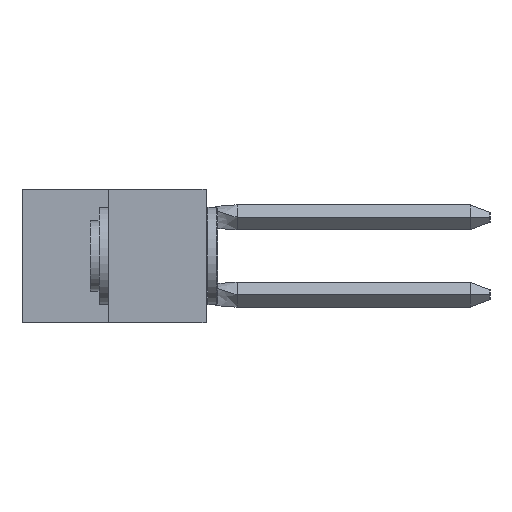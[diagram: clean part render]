
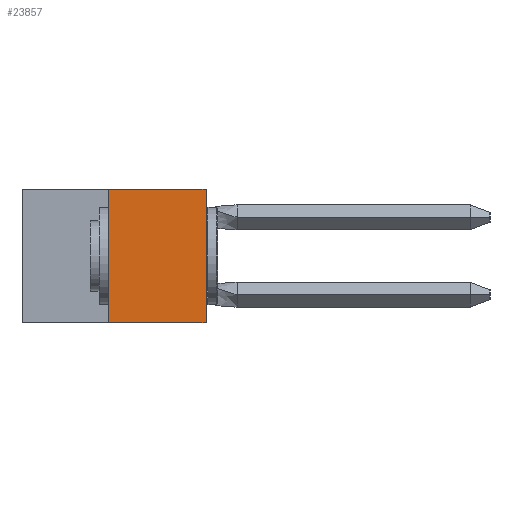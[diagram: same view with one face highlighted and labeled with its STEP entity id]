
A CAD part, left-side view. The second image highlights one B-rep face of the part: STEP entity #23857.
In plain terms, the highlighted planar face has unit normal (-1, 0, 0).
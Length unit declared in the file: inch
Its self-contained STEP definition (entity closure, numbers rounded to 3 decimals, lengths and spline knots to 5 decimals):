
#43 = PLANE ( 'NONE',  #45962 ) ;
#754 = EDGE_CURVE ( 'NONE', #29796, #30808, #2603, .T. ) ;
#1043 = LINE ( 'NONE', #20810, #19435 ) ;
#2603 = LINE ( 'NONE', #34126, #13179 ) ;
#4148 = ORIENTED_EDGE ( 'NONE', *, *, #39756, .T. ) ;
#5607 = DIRECTION ( 'NONE',  ( 0., 0., 1. ) ) ;
#7916 = DIRECTION ( 'NONE',  ( 0., 0., 1. ) ) ;
#8789 = VECTOR ( 'NONE', #33883, 39.37008 ) ;
#11732 = VERTEX_POINT ( 'NONE', #27683 ) ;
#11980 = EDGE_CURVE ( 'NONE', #30808, #11732, #1043, .T. ) ;
#13179 = VECTOR ( 'NONE', #5607, 39.37008 ) ;
#13882 = CARTESIAN_POINT ( 'NONE',  ( 0., 0.473, 0. ) ) ;
#14716 = VECTOR ( 'NONE', #7916, 39.37008 ) ;
#15080 = EDGE_CURVE ( 'NONE', #19869, #11732, #43048, .T. ) ;
#17890 = ORIENTED_EDGE ( 'NONE', *, *, #11980, .F. ) ;
#19435 = VECTOR ( 'NONE', #38668, 39.37008 ) ;
#19869 = VERTEX_POINT ( 'NONE', #27883 ) ;
#20692 = FACE_OUTER_BOUND ( 'NONE', #44973, .T. ) ;
#20810 = CARTESIAN_POINT ( 'NONE',  ( 0., 0.473, 0. ) ) ;
#21001 = LINE ( 'NONE', #37337, #8789 ) ;
#21902 = CARTESIAN_POINT ( 'NONE',  ( 0., 0., 0. ) ) ;
#23857 = ADVANCED_FACE ( 'NONE', ( #20692 ), #43, .F. ) ;
#24293 = DIRECTION ( 'NONE',  ( 1., 0., 0. ) ) ;
#26973 = ORIENTED_EDGE ( 'NONE', *, *, #15080, .T. ) ;
#27683 = CARTESIAN_POINT ( 'NONE',  ( 0., 0., 0. ) ) ;
#27883 = CARTESIAN_POINT ( 'NONE',  ( 0., 0., -0.343 ) ) ;
#29796 = VERTEX_POINT ( 'NONE', #35755 ) ;
#30808 = VERTEX_POINT ( 'NONE', #45371 ) ;
#31924 = ORIENTED_EDGE ( 'NONE', *, *, #754, .F. ) ;
#33883 = DIRECTION ( 'NONE',  ( 0., -1., 0. ) ) ;
#34126 = CARTESIAN_POINT ( 'NONE',  ( 0., 0.25, 0. ) ) ;
#35755 = CARTESIAN_POINT ( 'NONE',  ( 0., 0.25, -0.343 ) ) ;
#37337 = CARTESIAN_POINT ( 'NONE',  ( 0., 0.473, -0.343 ) ) ;
#38668 = DIRECTION ( 'NONE',  ( 0., -1., 0. ) ) ;
#39756 = EDGE_CURVE ( 'NONE', #29796, #19869, #21001, .T. ) ;
#43048 = LINE ( 'NONE', #21902, #14716 ) ;
#44973 = EDGE_LOOP ( 'NONE', ( #17890, #31924, #4148, #26973 ) ) ;
#45371 = CARTESIAN_POINT ( 'NONE',  ( 0., 0.25, 0. ) ) ;
#45867 = DIRECTION ( 'NONE',  ( 0., 0., -1. ) ) ;
#45962 = AXIS2_PLACEMENT_3D ( 'NONE', #13882, #24293, #45867 ) ;
